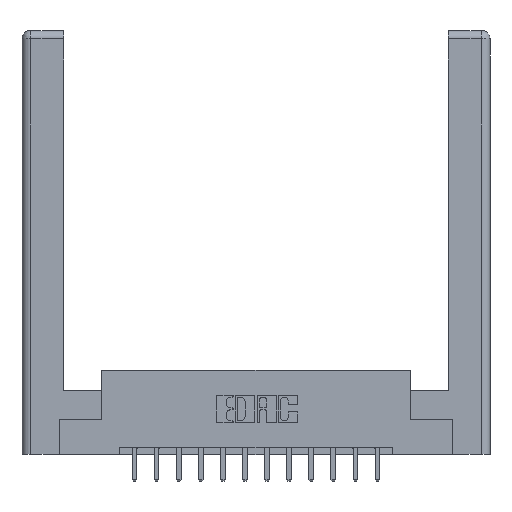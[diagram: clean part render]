
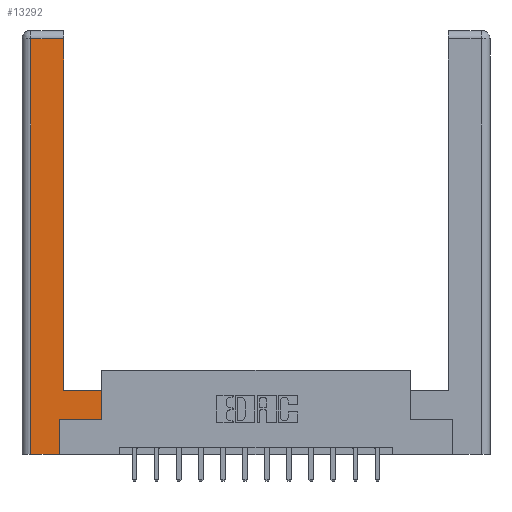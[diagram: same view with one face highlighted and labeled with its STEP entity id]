
A CAD part, top view. The second image highlights one B-rep face of the part: STEP entity #13292.
In plain terms, the highlighted planar face has unit normal (0, 0, 1).
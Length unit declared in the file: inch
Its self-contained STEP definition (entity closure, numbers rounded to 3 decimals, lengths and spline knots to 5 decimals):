
#258 = EDGE_CURVE ( 'NONE', #11812, #5372, #14517, .T. ) ;
#534 = EDGE_CURVE ( 'NONE', #7135, #2937, #5245, .T. ) ;
#548 = VECTOR ( 'NONE', #13333, 39.37008 ) ;
#830 = VERTEX_POINT ( 'NONE', #5057 ) ;
#1682 = FACE_OUTER_BOUND ( 'NONE', #4728, .T. ) ;
#1837 = EDGE_CURVE ( 'NONE', #12024, #7135, #2698, .T. ) ;
#1974 = EDGE_CURVE ( 'NONE', #5372, #12024, #12333, .T. ) ;
#2066 = CARTESIAN_POINT ( 'NONE',  ( 0.565, 0.45, 0. ) ) ;
#2090 = VERTEX_POINT ( 'NONE', #13550 ) ;
#2599 = DIRECTION ( 'NONE',  ( 0., -1., 0. ) ) ;
#2683 = ORIENTED_EDGE ( 'NONE', *, *, #1974, .T. ) ;
#2698 = LINE ( 'NONE', #10557, #12894 ) ;
#2740 = VECTOR ( 'NONE', #3411, 39.37008 ) ;
#2937 = VERTEX_POINT ( 'NONE', #4981 ) ;
#3411 = DIRECTION ( 'NONE',  ( 1., 0., 0. ) ) ;
#3499 = DIRECTION ( 'NONE',  ( -1., 0., 0. ) ) ;
#3521 = AXIS2_PLACEMENT_3D ( 'NONE', #12504, #8784, #4976 ) ;
#3809 = ORIENTED_EDGE ( 'NONE', *, *, #258, .T. ) ;
#3987 = LINE ( 'NONE', #2066, #9969 ) ;
#4602 = EDGE_CURVE ( 'NONE', #2937, #2090, #3987, .T. ) ;
#4728 = EDGE_LOOP ( 'NONE', ( #10023, #7504, #3809, #2683, #7172, #11762, #12628, #9216 ) ) ;
#4976 = DIRECTION ( 'NONE',  ( -1., 0., 0. ) ) ;
#4981 = CARTESIAN_POINT ( 'NONE',  ( 0.565, 0.245, 0. ) ) ;
#5057 = CARTESIAN_POINT ( 'NONE',  ( 0.295, 0.45, 0. ) ) ;
#5205 = LINE ( 'NONE', #7179, #13087 ) ;
#5228 = LINE ( 'NONE', #14671, #14070 ) ;
#5245 = LINE ( 'NONE', #10794, #2740 ) ;
#5372 = VERTEX_POINT ( 'NONE', #6473 ) ;
#5777 = CARTESIAN_POINT ( 'NONE',  ( 0.0615, 2.94, 0. ) ) ;
#5955 = DIRECTION ( 'NONE',  ( -1., 0., 0. ) ) ;
#6276 = VECTOR ( 'NONE', #5955, 39.37008 ) ;
#6473 = CARTESIAN_POINT ( 'NONE',  ( 0.0615, 0., 0. ) ) ;
#7135 = VERTEX_POINT ( 'NONE', #10701 ) ;
#7172 = ORIENTED_EDGE ( 'NONE', *, *, #1837, .T. ) ;
#7179 = CARTESIAN_POINT ( 'NONE',  ( 0.295, 0.45, 0. ) ) ;
#7470 = CARTESIAN_POINT ( 'NONE',  ( 0.0615, 0., 0. ) ) ;
#7504 = ORIENTED_EDGE ( 'NONE', *, *, #15449, .T. ) ;
#8784 = DIRECTION ( 'NONE',  ( 0., 0., -1. ) ) ;
#9216 = ORIENTED_EDGE ( 'NONE', *, *, #12576, .T. ) ;
#9293 = VERTEX_POINT ( 'NONE', #12121 ) ;
#9492 = DIRECTION ( 'NONE',  ( 0., 1., 0. ) ) ;
#9700 = DIRECTION ( 'NONE',  ( 0., 1., 0. ) ) ;
#9768 = PLANE ( 'NONE',  #3521 ) ;
#9969 = VECTOR ( 'NONE', #10672, 39.37008 ) ;
#10023 = ORIENTED_EDGE ( 'NONE', *, *, #11353, .T. ) ;
#10557 = CARTESIAN_POINT ( 'NONE',  ( 0.265, 0.245, 0. ) ) ;
#10672 = DIRECTION ( 'NONE',  ( 0., 1., 0. ) ) ;
#10701 = CARTESIAN_POINT ( 'NONE',  ( 0.265, 0.245, 0. ) ) ;
#10794 = CARTESIAN_POINT ( 'NONE',  ( 0.565, 0.245, 0. ) ) ;
#10857 = CARTESIAN_POINT ( 'NONE',  ( 0.0615, 2.94, 0. ) ) ;
#11353 = EDGE_CURVE ( 'NONE', #830, #9293, #5228, .T. ) ;
#11405 = CARTESIAN_POINT ( 'NONE',  ( 0.265, 0., 0. ) ) ;
#11762 = ORIENTED_EDGE ( 'NONE', *, *, #534, .T. ) ;
#11812 = VERTEX_POINT ( 'NONE', #5777 ) ;
#11843 = CARTESIAN_POINT ( 'NONE',  ( 0.265, 0., 0. ) ) ;
#12024 = VERTEX_POINT ( 'NONE', #11405 ) ;
#12121 = CARTESIAN_POINT ( 'NONE',  ( 0.295, 2.94, 0. ) ) ;
#12333 = LINE ( 'NONE', #11843, #548 ) ;
#12504 = CARTESIAN_POINT ( 'NONE',  ( 0., 0., 0. ) ) ;
#12576 = EDGE_CURVE ( 'NONE', #2090, #830, #5205, .T. ) ;
#12628 = ORIENTED_EDGE ( 'NONE', *, *, #4602, .T. ) ;
#12894 = VECTOR ( 'NONE', #9492, 39.37008 ) ;
#13087 = VECTOR ( 'NONE', #3499, 39.37008 ) ;
#13292 = ADVANCED_FACE ( 'NONE', ( #1682 ), #9768, .F. ) ;
#13333 = DIRECTION ( 'NONE',  ( 1., 0., 0. ) ) ;
#13550 = CARTESIAN_POINT ( 'NONE',  ( 0.565, 0.45, 0. ) ) ;
#14070 = VECTOR ( 'NONE', #9700, 39.37008 ) ;
#14517 = LINE ( 'NONE', #7470, #15077 ) ;
#14671 = CARTESIAN_POINT ( 'NONE',  ( 0.295, 3., 0. ) ) ;
#15077 = VECTOR ( 'NONE', #2599, 39.37008 ) ;
#15449 = EDGE_CURVE ( 'NONE', #9293, #11812, #15495, .T. ) ;
#15495 = LINE ( 'NONE', #10857, #6276 ) ;
